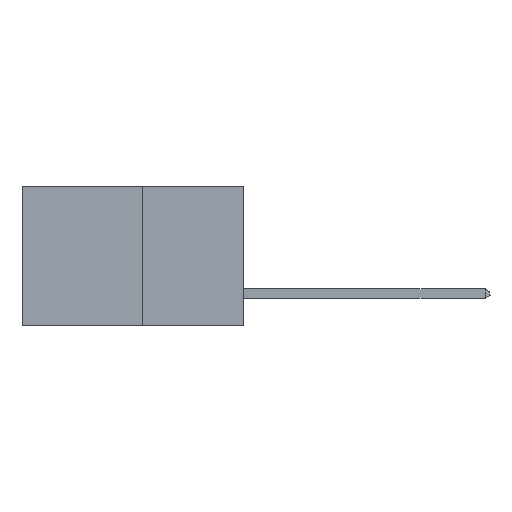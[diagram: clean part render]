
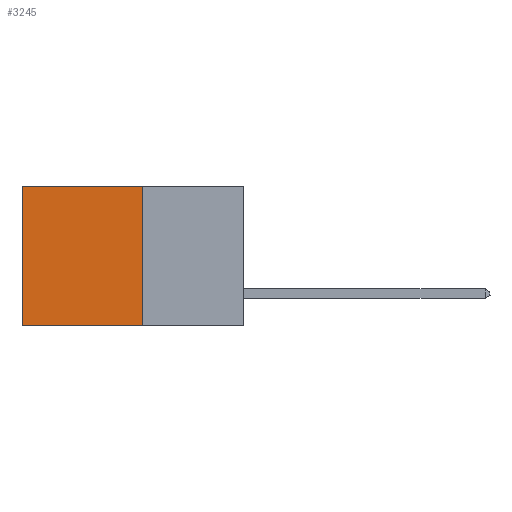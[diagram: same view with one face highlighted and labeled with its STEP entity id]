
A CAD part, left-side view. The second image highlights one B-rep face of the part: STEP entity #3245.
In plain terms, the highlighted planar face has unit normal (-1, 0, 0).
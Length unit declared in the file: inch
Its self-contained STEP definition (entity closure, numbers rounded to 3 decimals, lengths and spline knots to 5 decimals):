
#298 = EDGE_CURVE ( 'NONE', #4609, #3140, #6672, .T. ) ;
#978 = CARTESIAN_POINT ( 'NONE',  ( 0.277, 0.27, -0.37 ) ) ;
#1044 = FACE_OUTER_BOUND ( 'NONE', #12597, .T. ) ;
#1392 = VECTOR ( 'NONE', #12490, 39.37008 ) ;
#1483 = ORIENTED_EDGE ( 'NONE', *, *, #298, .T. ) ;
#1852 = CARTESIAN_POINT ( 'NONE',  ( 0.277, 0.27, -0.37 ) ) ;
#2756 = CARTESIAN_POINT ( 'NONE',  ( 0.277, 0.27, -0.37 ) ) ;
#2854 = DIRECTION ( 'NONE',  ( 0., 1., 0. ) ) ;
#3140 = VERTEX_POINT ( 'NONE', #3557 ) ;
#3141 = EDGE_CURVE ( 'NONE', #3321, #4609, #9790, .T. ) ;
#3245 = ADVANCED_FACE ( 'NONE', ( #1044 ), #9403, .F. ) ;
#3321 = VERTEX_POINT ( 'NONE', #8358 ) ;
#3422 = ORIENTED_EDGE ( 'NONE', *, *, #8341, .F. ) ;
#3557 = CARTESIAN_POINT ( 'NONE',  ( 0.277, 0.59, -0.37 ) ) ;
#3825 = CARTESIAN_POINT ( 'NONE',  ( 0.277, 0.27, 0. ) ) ;
#4029 = LINE ( 'NONE', #2756, #1392 ) ;
#4609 = VERTEX_POINT ( 'NONE', #5604 ) ;
#4636 = VECTOR ( 'NONE', #11994, 39.37008 ) ;
#4702 = VECTOR ( 'NONE', #2854, 39.37008 ) ;
#5255 = DIRECTION ( 'NONE',  ( 0., 0., -1. ) ) ;
#5359 = EDGE_CURVE ( 'NONE', #3321, #9608, #4029, .T. ) ;
#5604 = CARTESIAN_POINT ( 'NONE',  ( 0.277, 0.59, 0. ) ) ;
#6647 = DIRECTION ( 'NONE',  ( 1., 0., 0. ) ) ;
#6672 = LINE ( 'NONE', #9314, #9855 ) ;
#7273 = LINE ( 'NONE', #1852, #4702 ) ;
#7815 = DIRECTION ( 'NONE',  ( 0., 0., -1. ) ) ;
#8341 = EDGE_CURVE ( 'NONE', #9608, #3140, #7273, .T. ) ;
#8358 = CARTESIAN_POINT ( 'NONE',  ( 0.277, 0.27, 0. ) ) ;
#8541 = AXIS2_PLACEMENT_3D ( 'NONE', #12486, #6647, #5255 ) ;
#9314 = CARTESIAN_POINT ( 'NONE',  ( 0.277, 0.59, -0.37 ) ) ;
#9403 = PLANE ( 'NONE',  #8541 ) ;
#9608 = VERTEX_POINT ( 'NONE', #978 ) ;
#9787 = ORIENTED_EDGE ( 'NONE', *, *, #3141, .T. ) ;
#9790 = LINE ( 'NONE', #3825, #4636 ) ;
#9855 = VECTOR ( 'NONE', #7815, 39.37008 ) ;
#11994 = DIRECTION ( 'NONE',  ( 0., 1., 0. ) ) ;
#12176 = ORIENTED_EDGE ( 'NONE', *, *, #5359, .F. ) ;
#12486 = CARTESIAN_POINT ( 'NONE',  ( 0.277, 0.27, -0.37 ) ) ;
#12490 = DIRECTION ( 'NONE',  ( 0., 0., -1. ) ) ;
#12597 = EDGE_LOOP ( 'NONE', ( #1483, #3422, #12176, #9787 ) ) ;
